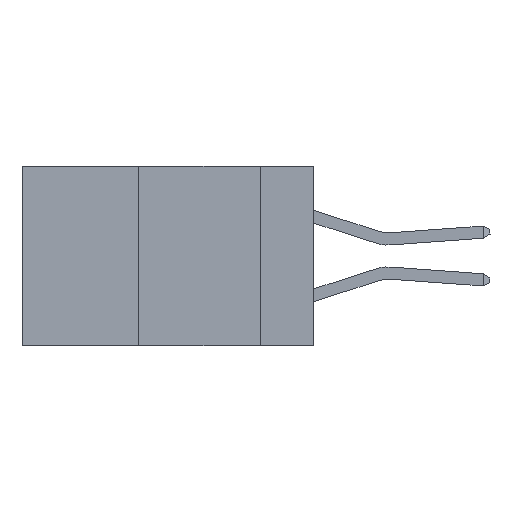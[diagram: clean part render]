
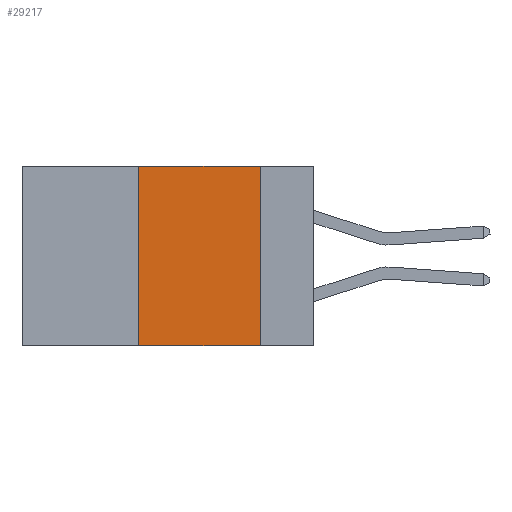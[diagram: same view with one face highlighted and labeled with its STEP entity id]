
A CAD part, left-side view. The second image highlights one B-rep face of the part: STEP entity #29217.
In plain terms, the highlighted planar face has unit normal (-1, 0, 0).
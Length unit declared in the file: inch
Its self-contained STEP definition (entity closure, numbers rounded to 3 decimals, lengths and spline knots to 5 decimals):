
#230 = VERTEX_POINT ( 'NONE', #4769 ) ;
#862 = CARTESIAN_POINT ( 'NONE',  ( 0., 0.11, 0. ) ) ;
#938 = EDGE_LOOP ( 'NONE', ( #15869, #11293, #31020, #44033 ) ) ;
#1774 = LINE ( 'NONE', #43387, #36874 ) ;
#3023 = DIRECTION ( 'NONE',  ( 0., 0., -1. ) ) ;
#3245 = LINE ( 'NONE', #33997, #36094 ) ;
#4659 = CARTESIAN_POINT ( 'NONE',  ( 0., 0.36, -0.37 ) ) ;
#4769 = CARTESIAN_POINT ( 'NONE',  ( 0., 0.11, -0.37 ) ) ;
#8540 = DIRECTION ( 'NONE',  ( 1., 0., 0. ) ) ;
#9454 = DIRECTION ( 'NONE',  ( 0., -1., 0. ) ) ;
#10638 = EDGE_CURVE ( 'NONE', #13654, #25079, #1774, .T. ) ;
#11293 = ORIENTED_EDGE ( 'NONE', *, *, #10638, .F. ) ;
#12362 = DIRECTION ( 'NONE',  ( 0., 0., -1. ) ) ;
#13654 = VERTEX_POINT ( 'NONE', #14089 ) ;
#14089 = CARTESIAN_POINT ( 'NONE',  ( 0., 0.36, 0. ) ) ;
#15869 = ORIENTED_EDGE ( 'NONE', *, *, #41498, .F. ) ;
#19127 = PLANE ( 'NONE',  #40461 ) ;
#20492 = LINE ( 'NONE', #26853, #43721 ) ;
#23119 = EDGE_CURVE ( 'NONE', #29591, #13654, #38980, .T. ) ;
#25079 = VERTEX_POINT ( 'NONE', #862 ) ;
#26853 = CARTESIAN_POINT ( 'NONE',  ( 0., 0.6, -0.37 ) ) ;
#28995 = CARTESIAN_POINT ( 'NONE',  ( 0., 0.36, 0. ) ) ;
#29217 = ADVANCED_FACE ( 'NONE', ( #36565 ), #19127, .F. ) ;
#29591 = VERTEX_POINT ( 'NONE', #4659 ) ;
#31020 = ORIENTED_EDGE ( 'NONE', *, *, #23119, .F. ) ;
#32393 = VECTOR ( 'NONE', #33059, 39.37008 ) ;
#33059 = DIRECTION ( 'NONE',  ( 0., 0., 1. ) ) ;
#33997 = CARTESIAN_POINT ( 'NONE',  ( 0., 0.11, 0. ) ) ;
#36094 = VECTOR ( 'NONE', #3023, 39.37008 ) ;
#36565 = FACE_OUTER_BOUND ( 'NONE', #938, .T. ) ;
#36639 = EDGE_CURVE ( 'NONE', #29591, #230, #20492, .T. ) ;
#36787 = CARTESIAN_POINT ( 'NONE',  ( 0., 0.6, 0. ) ) ;
#36874 = VECTOR ( 'NONE', #37034, 39.37008 ) ;
#37034 = DIRECTION ( 'NONE',  ( 0., -1., 0. ) ) ;
#38980 = LINE ( 'NONE', #28995, #32393 ) ;
#40461 = AXIS2_PLACEMENT_3D ( 'NONE', #36787, #8540, #12362 ) ;
#41498 = EDGE_CURVE ( 'NONE', #25079, #230, #3245, .T. ) ;
#43387 = CARTESIAN_POINT ( 'NONE',  ( 0., 0.6, 0. ) ) ;
#43721 = VECTOR ( 'NONE', #9454, 39.37008 ) ;
#44033 = ORIENTED_EDGE ( 'NONE', *, *, #36639, .T. ) ;
